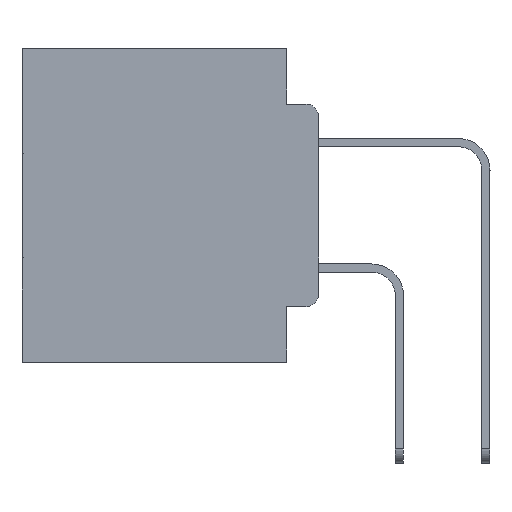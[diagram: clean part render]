
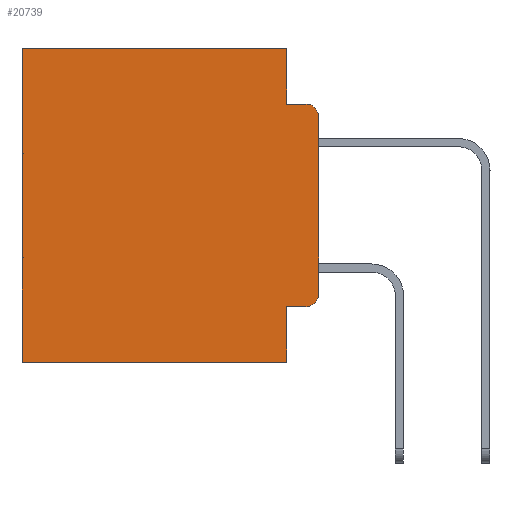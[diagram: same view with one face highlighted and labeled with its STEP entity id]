
A CAD part, left-side view. The second image highlights one B-rep face of the part: STEP entity #20739.
In plain terms, the highlighted planar face has unit normal (-1, 0, 0).
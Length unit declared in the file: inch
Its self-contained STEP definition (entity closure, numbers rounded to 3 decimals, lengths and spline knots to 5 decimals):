
#215 = DIRECTION ( 'NONE',  ( 0., 1., 0. ) ) ;
#2042 = CARTESIAN_POINT ( 'NONE',  ( 0.298, 0.02, -0.0885 ) ) ;
#2076 = EDGE_CURVE ( 'NONE', #25820, #22768, #3408, .T. ) ;
#3408 = CIRCLE ( 'NONE', #14534, 0.02 ) ;
#3747 = EDGE_CURVE ( 'NONE', #24384, #24222, #25669, .T. ) ;
#4292 = VERTEX_POINT ( 'NONE', #5285 ) ;
#4693 = EDGE_CURVE ( 'NONE', #12292, #24384, #22905, .T. ) ;
#4818 = DIRECTION ( 'NONE',  ( 0., -1., 0. ) ) ;
#5105 = CARTESIAN_POINT ( 'NONE',  ( 0.298, 0.02, -0.1085 ) ) ;
#5285 = CARTESIAN_POINT ( 'NONE',  ( 0.298, 0.051, 0. ) ) ;
#5310 = EDGE_CURVE ( 'NONE', #25820, #24222, #12617, .T. ) ;
#5550 = DIRECTION ( 'NONE',  ( 0., 0., -1. ) ) ;
#5662 = CARTESIAN_POINT ( 'NONE',  ( 0.298, 0.473, 0. ) ) ;
#5908 = DIRECTION ( 'NONE',  ( 0., 1., 0. ) ) ;
#5917 = VERTEX_POINT ( 'NONE', #8072 ) ;
#7109 = CARTESIAN_POINT ( 'NONE',  ( 0.298, 0.051, -0.0885 ) ) ;
#7246 = EDGE_CURVE ( 'NONE', #12292, #5917, #23636, .T. ) ;
#7819 = EDGE_CURVE ( 'NONE', #4292, #13485, #30428, .T. ) ;
#7964 = VECTOR ( 'NONE', #4818, 39.37008 ) ;
#8072 = CARTESIAN_POINT ( 'NONE',  ( 0.298, 0.051, -0.5 ) ) ;
#8299 = DIRECTION ( 'NONE',  ( 0., 0., -1. ) ) ;
#8362 = ORIENTED_EDGE ( 'NONE', *, *, #3747, .T. ) ;
#8742 = DIRECTION ( 'NONE',  ( 0., 0., -1. ) ) ;
#9083 = VECTOR ( 'NONE', #11990, 39.37008 ) ;
#9395 = LINE ( 'NONE', #27883, #32082 ) ;
#9692 = CARTESIAN_POINT ( 'NONE',  ( 0.298, 0.051, 0. ) ) ;
#9969 = CARTESIAN_POINT ( 'NONE',  ( 0.298, 0.051, -0.4115 ) ) ;
#10219 = EDGE_CURVE ( 'NONE', #13485, #22768, #28323, .T. ) ;
#10659 = CARTESIAN_POINT ( 'NONE',  ( 0.298, 0.051, -0.0885 ) ) ;
#11534 = DIRECTION ( 'NONE',  ( 0., 0., -1. ) ) ;
#11544 = VERTEX_POINT ( 'NONE', #29201 ) ;
#11990 = DIRECTION ( 'NONE',  ( 0., 0., -1. ) ) ;
#12057 = VECTOR ( 'NONE', #11534, 39.37008 ) ;
#12292 = VERTEX_POINT ( 'NONE', #28717 ) ;
#12310 = ORIENTED_EDGE ( 'NONE', *, *, #31031, .F. ) ;
#12565 = EDGE_CURVE ( 'NONE', #4292, #23013, #9395, .T. ) ;
#12617 = LINE ( 'NONE', #26161, #21266 ) ;
#13177 = DIRECTION ( 'NONE',  ( 0., -1., 0. ) ) ;
#13485 = VERTEX_POINT ( 'NONE', #7109 ) ;
#13587 = ORIENTED_EDGE ( 'NONE', *, *, #12565, .T. ) ;
#14534 = AXIS2_PLACEMENT_3D ( 'NONE', #5105, #25470, #22999 ) ;
#14834 = LINE ( 'NONE', #30324, #27346 ) ;
#16078 = EDGE_CURVE ( 'NONE', #23013, #11544, #17870, .T. ) ;
#16272 = ORIENTED_EDGE ( 'NONE', *, *, #7246, .F. ) ;
#17071 = ORIENTED_EDGE ( 'NONE', *, *, #4693, .T. ) ;
#17870 = LINE ( 'NONE', #5662, #25699 ) ;
#18830 = ORIENTED_EDGE ( 'NONE', *, *, #10219, .F. ) ;
#19514 = AXIS2_PLACEMENT_3D ( 'NONE', #20945, #30814, #8299 ) ;
#20739 = ADVANCED_FACE ( 'NONE', ( #27506 ), #28531, .F. ) ;
#20945 = CARTESIAN_POINT ( 'NONE',  ( 0.298, 0., 0. ) ) ;
#21266 = VECTOR ( 'NONE', #8742, 39.37008 ) ;
#21505 = ORIENTED_EDGE ( 'NONE', *, *, #2076, .T. ) ;
#22433 = DIRECTION ( 'NONE',  ( 0., 0., -1. ) ) ;
#22768 = VERTEX_POINT ( 'NONE', #2042 ) ;
#22836 = EDGE_LOOP ( 'NONE', ( #27004, #21505, #18830, #29742, #13587, #32106, #12310, #16272, #17071, #8362 ) ) ;
#22905 = LINE ( 'NONE', #9969, #7964 ) ;
#22999 = DIRECTION ( 'NONE',  ( 0., 0., -1. ) ) ;
#23013 = VERTEX_POINT ( 'NONE', #25885 ) ;
#23091 = CARTESIAN_POINT ( 'NONE',  ( 0.298, 0., -0.1085 ) ) ;
#23636 = LINE ( 'NONE', #9692, #9083 ) ;
#24222 = VERTEX_POINT ( 'NONE', #28735 ) ;
#24384 = VERTEX_POINT ( 'NONE', #29281 ) ;
#24688 = DIRECTION ( 'NONE',  ( -1., 0., 0. ) ) ;
#25470 = DIRECTION ( 'NONE',  ( -1., 0., 0. ) ) ;
#25669 = CIRCLE ( 'NONE', #30657, 0.02 ) ;
#25699 = VECTOR ( 'NONE', #5550, 39.37008 ) ;
#25820 = VERTEX_POINT ( 'NONE', #23091 ) ;
#25885 = CARTESIAN_POINT ( 'NONE',  ( 0.298, 0.473, 0. ) ) ;
#26161 = CARTESIAN_POINT ( 'NONE',  ( 0.298, 0., 0. ) ) ;
#26849 = CARTESIAN_POINT ( 'NONE',  ( 0.298, 0.02, -0.3915 ) ) ;
#27004 = ORIENTED_EDGE ( 'NONE', *, *, #5310, .F. ) ;
#27346 = VECTOR ( 'NONE', #5908, 39.37008 ) ;
#27506 = FACE_OUTER_BOUND ( 'NONE', #22836, .T. ) ;
#27883 = CARTESIAN_POINT ( 'NONE',  ( 0.298, 0., 0. ) ) ;
#28323 = LINE ( 'NONE', #10659, #32234 ) ;
#28531 = PLANE ( 'NONE',  #19514 ) ;
#28717 = CARTESIAN_POINT ( 'NONE',  ( 0.298, 0.051, -0.4115 ) ) ;
#28735 = CARTESIAN_POINT ( 'NONE',  ( 0.298, 0., -0.3915 ) ) ;
#29201 = CARTESIAN_POINT ( 'NONE',  ( 0.298, 0.473, -0.5 ) ) ;
#29281 = CARTESIAN_POINT ( 'NONE',  ( 0.298, 0.02, -0.4115 ) ) ;
#29742 = ORIENTED_EDGE ( 'NONE', *, *, #7819, .F. ) ;
#30324 = CARTESIAN_POINT ( 'NONE',  ( 0.298, 0., -0.5 ) ) ;
#30428 = LINE ( 'NONE', #31419, #12057 ) ;
#30657 = AXIS2_PLACEMENT_3D ( 'NONE', #26849, #24688, #22433 ) ;
#30814 = DIRECTION ( 'NONE',  ( 1., 0., 0. ) ) ;
#31031 = EDGE_CURVE ( 'NONE', #5917, #11544, #14834, .T. ) ;
#31419 = CARTESIAN_POINT ( 'NONE',  ( 0.298, 0.051, 0. ) ) ;
#32082 = VECTOR ( 'NONE', #215, 39.37008 ) ;
#32106 = ORIENTED_EDGE ( 'NONE', *, *, #16078, .T. ) ;
#32234 = VECTOR ( 'NONE', #13177, 39.37008 ) ;
